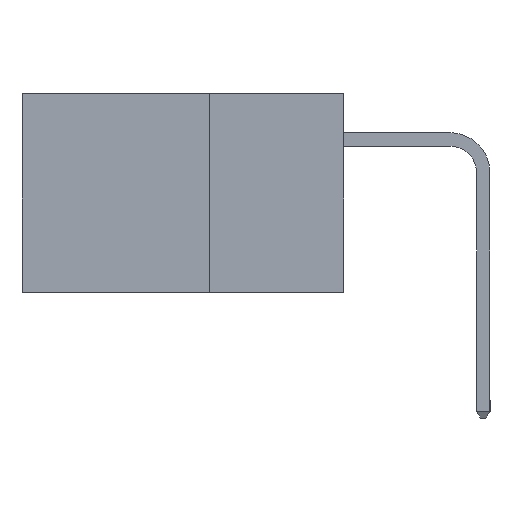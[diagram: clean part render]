
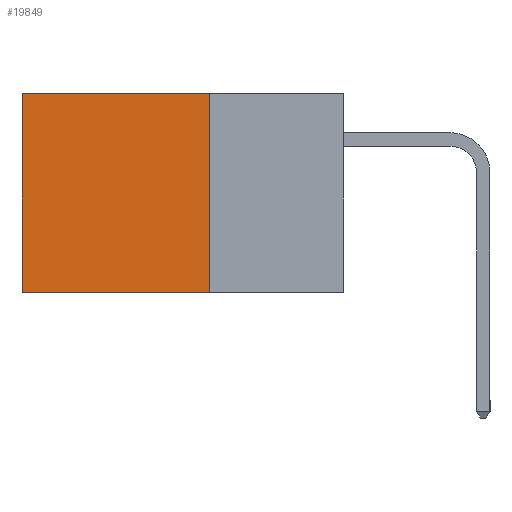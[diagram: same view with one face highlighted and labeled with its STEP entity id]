
A CAD part, left-side view. The second image highlights one B-rep face of the part: STEP entity #19849.
In plain terms, the highlighted planar face has unit normal (-1, 0, 0).
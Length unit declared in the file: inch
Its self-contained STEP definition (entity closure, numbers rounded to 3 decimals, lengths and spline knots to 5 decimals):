
#30 = VERTEX_POINT ( 'NONE', #20172 ) ;
#61 = LINE ( 'NONE', #2143, #21274 ) ;
#1107 = VERTEX_POINT ( 'NONE', #11881 ) ;
#2014 = DIRECTION ( 'NONE',  ( 0., 0., -1. ) ) ;
#2143 = CARTESIAN_POINT ( 'NONE',  ( 0.2615, 0.25, -0.37 ) ) ;
#2398 = DIRECTION ( 'NONE',  ( 1., 0., 0. ) ) ;
#5561 = VECTOR ( 'NONE', #2014, 39.37008 ) ;
#6015 = ORIENTED_EDGE ( 'NONE', *, *, #9078, .F. ) ;
#6025 = DIRECTION ( 'NONE',  ( 0., 1., 0. ) ) ;
#6376 = PLANE ( 'NONE',  #9645 ) ;
#7372 = EDGE_LOOP ( 'NONE', ( #25492, #6015, #18914, #13919 ) ) ;
#9078 = EDGE_CURVE ( 'NONE', #18063, #30, #61, .T. ) ;
#9645 = AXIS2_PLACEMENT_3D ( 'NONE', #14413, #2398, #16385 ) ;
#10146 = VECTOR ( 'NONE', #15696, 39.37008 ) ;
#11386 = LINE ( 'NONE', #17933, #16611 ) ;
#11881 = CARTESIAN_POINT ( 'NONE',  ( 0.2615, 0.6, 0. ) ) ;
#12939 = CARTESIAN_POINT ( 'NONE',  ( 0.2615, 0.25, -0.37 ) ) ;
#13919 = ORIENTED_EDGE ( 'NONE', *, *, #14554, .T. ) ;
#14413 = CARTESIAN_POINT ( 'NONE',  ( 0.2615, 0.25, -0.37 ) ) ;
#14554 = EDGE_CURVE ( 'NONE', #19750, #1107, #11386, .T. ) ;
#15394 = LINE ( 'NONE', #19577, #10146 ) ;
#15696 = DIRECTION ( 'NONE',  ( 0., 0., -1. ) ) ;
#16151 = DIRECTION ( 'NONE',  ( 0., 1., 0. ) ) ;
#16385 = DIRECTION ( 'NONE',  ( 0., 0., -1. ) ) ;
#16493 = EDGE_CURVE ( 'NONE', #1107, #30, #16772, .T. ) ;
#16611 = VECTOR ( 'NONE', #6025, 39.37008 ) ;
#16772 = LINE ( 'NONE', #23401, #5561 ) ;
#17933 = CARTESIAN_POINT ( 'NONE',  ( 0.2615, 0.25, 0. ) ) ;
#18063 = VERTEX_POINT ( 'NONE', #12939 ) ;
#18914 = ORIENTED_EDGE ( 'NONE', *, *, #19649, .F. ) ;
#19577 = CARTESIAN_POINT ( 'NONE',  ( 0.2615, 0.25, -0.37 ) ) ;
#19649 = EDGE_CURVE ( 'NONE', #19750, #18063, #15394, .T. ) ;
#19750 = VERTEX_POINT ( 'NONE', #21861 ) ;
#19849 = ADVANCED_FACE ( 'NONE', ( #25496 ), #6376, .F. ) ;
#20172 = CARTESIAN_POINT ( 'NONE',  ( 0.2615, 0.6, -0.37 ) ) ;
#21274 = VECTOR ( 'NONE', #16151, 39.37008 ) ;
#21861 = CARTESIAN_POINT ( 'NONE',  ( 0.2615, 0.25, 0. ) ) ;
#23401 = CARTESIAN_POINT ( 'NONE',  ( 0.2615, 0.6, -0.37 ) ) ;
#25492 = ORIENTED_EDGE ( 'NONE', *, *, #16493, .T. ) ;
#25496 = FACE_OUTER_BOUND ( 'NONE', #7372, .T. ) ;
